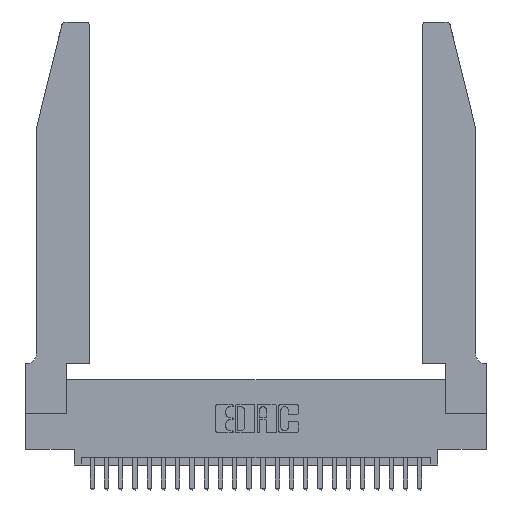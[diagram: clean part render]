
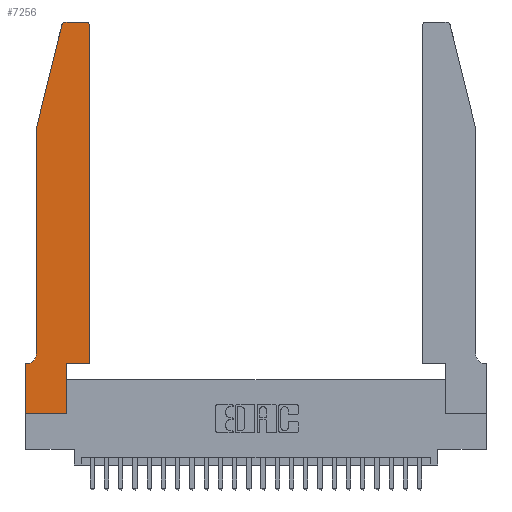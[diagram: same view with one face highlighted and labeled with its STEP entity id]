
A CAD part, top view. The second image highlights one B-rep face of the part: STEP entity #7256.
In plain terms, the highlighted planar face has unit normal (0, 0, 1).
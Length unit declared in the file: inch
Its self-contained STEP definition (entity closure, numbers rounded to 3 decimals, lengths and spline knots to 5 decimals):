
#154 = DIRECTION ( 'NONE',  ( 0., 0., 1. ) ) ;
#705 = CARTESIAN_POINT ( 'NONE',  ( 0.284, 2.72, 0.37 ) ) ;
#843 = CARTESIAN_POINT ( 'NONE',  ( 0.2865, 0.35, 0.37 ) ) ;
#1046 = VECTOR ( 'NONE', #2006, 39.37008 ) ;
#1276 = PLANE ( 'NONE',  #23185 ) ;
#1395 = VECTOR ( 'NONE', #14707, 39.37008 ) ;
#1589 = EDGE_CURVE ( 'NONE', #24942, #7070, #24709, .T. ) ;
#1654 = AXIS2_PLACEMENT_3D ( 'NONE', #12356, #154, #14464 ) ;
#1832 = EDGE_CURVE ( 'NONE', #8041, #4282, #8825, .T. ) ;
#1836 = FACE_OUTER_BOUND ( 'NONE', #5560, .T. ) ;
#1913 = ORIENTED_EDGE ( 'NONE', *, *, #17264, .T. ) ;
#2006 = DIRECTION ( 'NONE',  ( 0., -1., 0. ) ) ;
#2186 = CARTESIAN_POINT ( 'NONE',  ( 0., 0., 0.37 ) ) ;
#2350 = EDGE_CURVE ( 'NONE', #15674, #22785, #13593, .T. ) ;
#3129 = VECTOR ( 'NONE', #23273, 39.37008 ) ;
#3222 = VECTOR ( 'NONE', #11413, 39.37008 ) ;
#3336 = DIRECTION ( 'NONE',  ( 1., 0., 0. ) ) ;
#3515 = AXIS2_PLACEMENT_3D ( 'NONE', #705, #11788, #3564 ) ;
#3564 = DIRECTION ( 'NONE',  ( 1., 0., 0. ) ) ;
#4282 = VERTEX_POINT ( 'NONE', #5957 ) ;
#4303 = AXIS2_PLACEMENT_3D ( 'NONE', #22755, #10543, #24742 ) ;
#5168 = LINE ( 'NONE', #13247, #15405 ) ;
#5433 = CARTESIAN_POINT ( 'NONE',  ( 0., 0.35, 0.37 ) ) ;
#5545 = VECTOR ( 'NONE', #12323, 39.37008 ) ;
#5560 = EDGE_LOOP ( 'NONE', ( #11232, #9411, #1913, #12671, #17018, #10399, #14073, #14042, #16498, #15888, #9638, #9233 ) ) ;
#5957 = CARTESIAN_POINT ( 'NONE',  ( 0.25487, 2.72718, 0.37 ) ) ;
#6599 = VECTOR ( 'NONE', #16829, 39.37008 ) ;
#6692 = CARTESIAN_POINT ( 'NONE',  ( 0., 0., 0.37 ) ) ;
#6834 = CARTESIAN_POINT ( 'NONE',  ( 0.4505, 2.72, 0.37 ) ) ;
#6879 = VECTOR ( 'NONE', #21552, 39.37008 ) ;
#6900 = DIRECTION ( 'NONE',  ( 0., 1., 0. ) ) ;
#7070 = VERTEX_POINT ( 'NONE', #21119 ) ;
#7256 = ADVANCED_FACE ( 'NONE', ( #1836 ), #1276, .T. ) ;
#7316 = CARTESIAN_POINT ( 'NONE',  ( 0., 0.35, 0.37 ) ) ;
#7627 = CARTESIAN_POINT ( 'NONE',  ( 0.4505, 0.35, 0.37 ) ) ;
#8041 = VERTEX_POINT ( 'NONE', #8277 ) ;
#8277 = CARTESIAN_POINT ( 'NONE',  ( 0.284, 2.75, 0.37 ) ) ;
#8627 = LINE ( 'NONE', #9363, #3222 ) ;
#8642 = EDGE_CURVE ( 'NONE', #20794, #15674, #18716, .T. ) ;
#8796 = EDGE_CURVE ( 'NONE', #7070, #9197, #25547, .T. ) ;
#8825 = CIRCLE ( 'NONE', #3515, 0.03 ) ;
#9078 = CARTESIAN_POINT ( 'NONE',  ( 0.0755, 2., 0.37 ) ) ;
#9197 = VERTEX_POINT ( 'NONE', #14217 ) ;
#9233 = ORIENTED_EDGE ( 'NONE', *, *, #16943, .T. ) ;
#9363 = CARTESIAN_POINT ( 'NONE',  ( 0.2605, 2.75, 0.37 ) ) ;
#9391 = CARTESIAN_POINT ( 'NONE',  ( 0.4205, 2.75, 0.37 ) ) ;
#9411 = ORIENTED_EDGE ( 'NONE', *, *, #1832, .T. ) ;
#9638 = ORIENTED_EDGE ( 'NONE', *, *, #13769, .T. ) ;
#10266 = CARTESIAN_POINT ( 'NONE',  ( 0.0755, 2., 0.37 ) ) ;
#10399 = ORIENTED_EDGE ( 'NONE', *, *, #2350, .T. ) ;
#10543 = DIRECTION ( 'NONE',  ( 0., 0., -1. ) ) ;
#11232 = ORIENTED_EDGE ( 'NONE', *, *, #21591, .T. ) ;
#11413 = DIRECTION ( 'NONE',  ( -1., 0., 0. ) ) ;
#11788 = DIRECTION ( 'NONE',  ( 0., 0., 1. ) ) ;
#11826 = VERTEX_POINT ( 'NONE', #9078 ) ;
#11868 = LINE ( 'NONE', #26249, #1046 ) ;
#12218 = LINE ( 'NONE', #12596, #1395 ) ;
#12323 = DIRECTION ( 'NONE',  ( 0., -1., 0. ) ) ;
#12356 = CARTESIAN_POINT ( 'NONE',  ( 0.4205, 2.72, 0.37 ) ) ;
#12451 = CARTESIAN_POINT ( 'NONE',  ( 0.0755, 0.42, 0.37 ) ) ;
#12595 = CARTESIAN_POINT ( 'NONE',  ( 0.0055, 0.35, 0.37 ) ) ;
#12596 = CARTESIAN_POINT ( 'NONE',  ( 0.4505, 0.35, 0.37 ) ) ;
#12671 = ORIENTED_EDGE ( 'NONE', *, *, #26042, .T. ) ;
#13247 = CARTESIAN_POINT ( 'NONE',  ( 0.0755, 2., 0.37 ) ) ;
#13593 = LINE ( 'NONE', #18560, #6879 ) ;
#13769 = EDGE_CURVE ( 'NONE', #16739, #19226, #22836, .T. ) ;
#14042 = ORIENTED_EDGE ( 'NONE', *, *, #1589, .T. ) ;
#14073 = ORIENTED_EDGE ( 'NONE', *, *, #16212, .T. ) ;
#14217 = CARTESIAN_POINT ( 'NONE',  ( 0.2865, 0.35, 0.37 ) ) ;
#14464 = DIRECTION ( 'NONE',  ( 1., 0., 0. ) ) ;
#14707 = DIRECTION ( 'NONE',  ( 1., 0., 0. ) ) ;
#14722 = CARTESIAN_POINT ( 'NONE',  ( 0.4505, 0.35, 0.37 ) ) ;
#15365 = DIRECTION ( 'NONE',  ( -0.239, -0.971, 0. ) ) ;
#15405 = VECTOR ( 'NONE', #15365, 39.37008 ) ;
#15600 = DIRECTION ( 'NONE',  ( 0., 0., 1. ) ) ;
#15674 = VERTEX_POINT ( 'NONE', #12595 ) ;
#15888 = ORIENTED_EDGE ( 'NONE', *, *, #19797, .T. ) ;
#16212 = EDGE_CURVE ( 'NONE', #22785, #24942, #11868, .T. ) ;
#16498 = ORIENTED_EDGE ( 'NONE', *, *, #8796, .T. ) ;
#16739 = VERTEX_POINT ( 'NONE', #7627 ) ;
#16829 = DIRECTION ( 'NONE',  ( 0., 1., 0. ) ) ;
#16943 = EDGE_CURVE ( 'NONE', #19226, #25746, #22995, .T. ) ;
#17018 = ORIENTED_EDGE ( 'NONE', *, *, #8642, .T. ) ;
#17109 = LINE ( 'NONE', #10266, #5545 ) ;
#17264 = EDGE_CURVE ( 'NONE', #4282, #11826, #5168, .T. ) ;
#18560 = CARTESIAN_POINT ( 'NONE',  ( 0.0755, 0.35, 0.37 ) ) ;
#18716 = CIRCLE ( 'NONE', #4303, 0.07 ) ;
#19226 = VERTEX_POINT ( 'NONE', #6834 ) ;
#19797 = EDGE_CURVE ( 'NONE', #9197, #16739, #12218, .T. ) ;
#20794 = VERTEX_POINT ( 'NONE', #12451 ) ;
#20915 = VECTOR ( 'NONE', #6900, 39.37008 ) ;
#21119 = CARTESIAN_POINT ( 'NONE',  ( 0.2865, 0., 0.37 ) ) ;
#21552 = DIRECTION ( 'NONE',  ( -1., 0., 0. ) ) ;
#21591 = EDGE_CURVE ( 'NONE', #25746, #8041, #8627, .T. ) ;
#22755 = CARTESIAN_POINT ( 'NONE',  ( 0.0055, 0.42, 0.37 ) ) ;
#22785 = VERTEX_POINT ( 'NONE', #5433 ) ;
#22836 = LINE ( 'NONE', #14722, #6599 ) ;
#22995 = CIRCLE ( 'NONE', #1654, 0.03 ) ;
#23185 = AXIS2_PLACEMENT_3D ( 'NONE', #7316, #15600, #3336 ) ;
#23273 = DIRECTION ( 'NONE',  ( 1., 0., 0. ) ) ;
#24709 = LINE ( 'NONE', #2186, #3129 ) ;
#24742 = DIRECTION ( 'NONE',  ( -1., 0., 0. ) ) ;
#24942 = VERTEX_POINT ( 'NONE', #6692 ) ;
#25547 = LINE ( 'NONE', #843, #20915 ) ;
#25746 = VERTEX_POINT ( 'NONE', #9391 ) ;
#26042 = EDGE_CURVE ( 'NONE', #11826, #20794, #17109, .T. ) ;
#26249 = CARTESIAN_POINT ( 'NONE',  ( 0., 0., 0.37 ) ) ;
